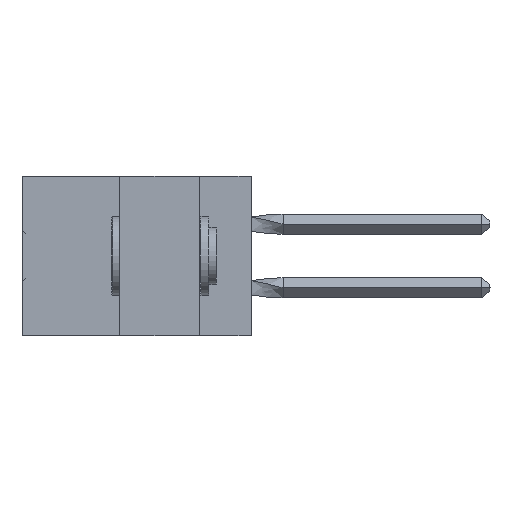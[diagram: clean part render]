
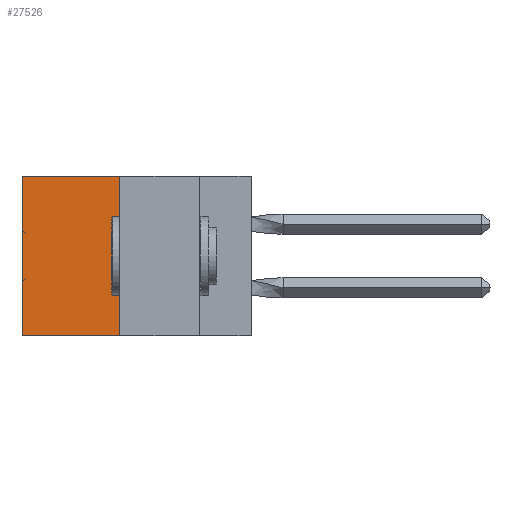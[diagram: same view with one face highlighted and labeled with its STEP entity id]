
A CAD part, left-side view. The second image highlights one B-rep face of the part: STEP entity #27526.
In plain terms, the highlighted planar face has unit normal (-1, 0, 0).
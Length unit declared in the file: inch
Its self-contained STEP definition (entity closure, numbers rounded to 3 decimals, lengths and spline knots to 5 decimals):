
#3455 = EDGE_CURVE ( 'NONE', #34702, #54368, #10836, .T. ) ;
#4919 = CARTESIAN_POINT ( 'NONE',  ( 0.305, 0.72, -0.5 ) ) ;
#5106 = CARTESIAN_POINT ( 'NONE',  ( 0.305, 0.413, -0.5 ) ) ;
#6339 = LINE ( 'NONE', #10930, #52359 ) ;
#6757 = FACE_OUTER_BOUND ( 'NONE', #40337, .T. ) ;
#8613 = LINE ( 'NONE', #5106, #51799 ) ;
#9696 = ORIENTED_EDGE ( 'NONE', *, *, #3455, .F. ) ;
#10569 = CARTESIAN_POINT ( 'NONE',  ( 0.305, 0.413, -0.5 ) ) ;
#10836 = LINE ( 'NONE', #10569, #44119 ) ;
#10930 = CARTESIAN_POINT ( 'NONE',  ( 0.305, 0.413, 0. ) ) ;
#14284 = CARTESIAN_POINT ( 'NONE',  ( 0.305, 0.72, 0. ) ) ;
#17391 = EDGE_CURVE ( 'NONE', #57744, #34702, #8613, .T. ) ;
#20937 = CARTESIAN_POINT ( 'NONE',  ( 0.305, 0.413, -0.5 ) ) ;
#24273 = DIRECTION ( 'NONE',  ( 0., 1., 0. ) ) ;
#25171 = CARTESIAN_POINT ( 'NONE',  ( 0.305, 0.413, 0. ) ) ;
#27526 = ADVANCED_FACE ( 'NONE', ( #6757 ), #43071, .F. ) ;
#29202 = EDGE_CURVE ( 'NONE', #57744, #47795, #6339, .T. ) ;
#29552 = DIRECTION ( 'NONE',  ( 0., 0., -1. ) ) ;
#30813 = LINE ( 'NONE', #4919, #35078 ) ;
#31732 = CARTESIAN_POINT ( 'NONE',  ( 0.305, 0.413, -0.5 ) ) ;
#33520 = CARTESIAN_POINT ( 'NONE',  ( 0.305, 0.72, -0.5 ) ) ;
#34702 = VERTEX_POINT ( 'NONE', #31732 ) ;
#35078 = VECTOR ( 'NONE', #54270, 39.37008 ) ;
#37327 = DIRECTION ( 'NONE',  ( 1., 0., 0. ) ) ;
#37475 = EDGE_CURVE ( 'NONE', #47795, #54368, #30813, .T. ) ;
#40337 = EDGE_LOOP ( 'NONE', ( #52889, #9696, #50026, #50240 ) ) ;
#42607 = DIRECTION ( 'NONE',  ( 0., 1., 0. ) ) ;
#43071 = PLANE ( 'NONE',  #46276 ) ;
#44119 = VECTOR ( 'NONE', #24273, 39.37008 ) ;
#46276 = AXIS2_PLACEMENT_3D ( 'NONE', #20937, #37327, #57127 ) ;
#47795 = VERTEX_POINT ( 'NONE', #14284 ) ;
#50026 = ORIENTED_EDGE ( 'NONE', *, *, #17391, .F. ) ;
#50240 = ORIENTED_EDGE ( 'NONE', *, *, #29202, .T. ) ;
#51799 = VECTOR ( 'NONE', #29552, 39.37008 ) ;
#52359 = VECTOR ( 'NONE', #42607, 39.37008 ) ;
#52889 = ORIENTED_EDGE ( 'NONE', *, *, #37475, .T. ) ;
#54270 = DIRECTION ( 'NONE',  ( 0., 0., -1. ) ) ;
#54368 = VERTEX_POINT ( 'NONE', #33520 ) ;
#57127 = DIRECTION ( 'NONE',  ( 0., 0., -1. ) ) ;
#57744 = VERTEX_POINT ( 'NONE', #25171 ) ;
